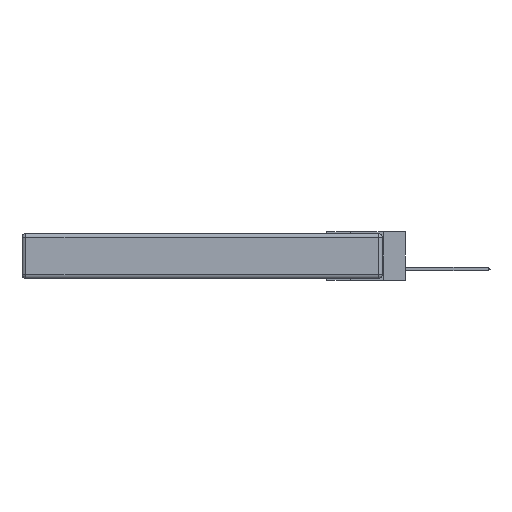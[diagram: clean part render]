
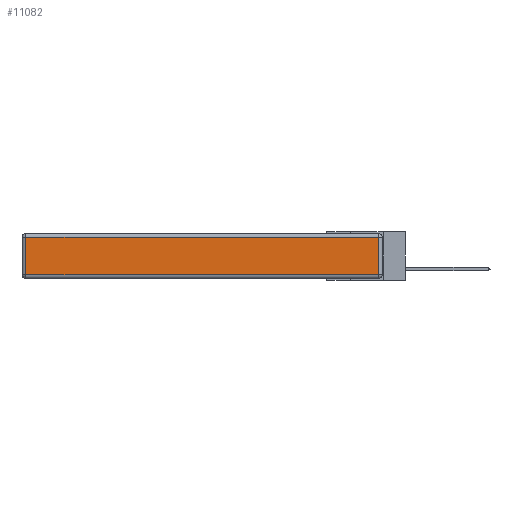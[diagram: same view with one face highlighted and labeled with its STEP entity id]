
A CAD part, left-side view. The second image highlights one B-rep face of the part: STEP entity #11082.
In plain terms, the highlighted planar face has unit normal (-1, 0, 0).
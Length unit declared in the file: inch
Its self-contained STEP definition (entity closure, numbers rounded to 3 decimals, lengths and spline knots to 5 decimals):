
#21 = EDGE_CURVE ( 'NONE', #5914, #2844, #9490, .T. ) ;
#1208 = ORIENTED_EDGE ( 'NONE', *, *, #21, .T. ) ;
#1388 = EDGE_CURVE ( 'NONE', #2844, #13567, #2982, .T. ) ;
#2119 = CARTESIAN_POINT ( 'NONE',  ( 0., 2.75, -0.03 ) ) ;
#2769 = DIRECTION ( 'NONE',  ( 0., 0., -1. ) ) ;
#2844 = VERTEX_POINT ( 'NONE', #3910 ) ;
#2982 = LINE ( 'NONE', #2119, #16490 ) ;
#3050 = DIRECTION ( 'NONE',  ( 0., -1., 0. ) ) ;
#3910 = CARTESIAN_POINT ( 'NONE',  ( 0., 0.03, -0.03 ) ) ;
#3968 = EDGE_CURVE ( 'NONE', #13567, #10532, #14343, .T. ) ;
#4058 = EDGE_CURVE ( 'NONE', #10532, #5914, #4957, .T. ) ;
#4348 = ORIENTED_EDGE ( 'NONE', *, *, #1388, .T. ) ;
#4957 = LINE ( 'NONE', #16259, #12901 ) ;
#5750 = DIRECTION ( 'NONE',  ( 0., 0., 1. ) ) ;
#5789 = DIRECTION ( 'NONE',  ( 0., 0., 1. ) ) ;
#5914 = VERTEX_POINT ( 'NONE', #15544 ) ;
#6654 = CARTESIAN_POINT ( 'NONE',  ( 0., 2.72, -0.343 ) ) ;
#7265 = CARTESIAN_POINT ( 'NONE',  ( 0., 2.72, -0.03 ) ) ;
#8497 = PLANE ( 'NONE',  #8661 ) ;
#8611 = DIRECTION ( 'NONE',  ( -1., 0., 0. ) ) ;
#8661 = AXIS2_PLACEMENT_3D ( 'NONE', #13619, #8611, #5789 ) ;
#9490 = LINE ( 'NONE', #16278, #13203 ) ;
#10532 = VERTEX_POINT ( 'NONE', #13823 ) ;
#11082 = ADVANCED_FACE ( 'NONE', ( #13714 ), #8497, .T. ) ;
#11393 = ORIENTED_EDGE ( 'NONE', *, *, #4058, .T. ) ;
#12901 = VECTOR ( 'NONE', #3050, 39.37008 ) ;
#13203 = VECTOR ( 'NONE', #5750, 39.37008 ) ;
#13567 = VERTEX_POINT ( 'NONE', #7265 ) ;
#13619 = CARTESIAN_POINT ( 'NONE',  ( 0., 0., -0.343 ) ) ;
#13714 = FACE_OUTER_BOUND ( 'NONE', #15087, .T. ) ;
#13782 = DIRECTION ( 'NONE',  ( 0., 1., 0. ) ) ;
#13823 = CARTESIAN_POINT ( 'NONE',  ( 0., 2.72, -0.313 ) ) ;
#14317 = VECTOR ( 'NONE', #2769, 39.37008 ) ;
#14343 = LINE ( 'NONE', #6654, #14317 ) ;
#14547 = ORIENTED_EDGE ( 'NONE', *, *, #3968, .T. ) ;
#15087 = EDGE_LOOP ( 'NONE', ( #11393, #1208, #4348, #14547 ) ) ;
#15544 = CARTESIAN_POINT ( 'NONE',  ( 0., 0.03, -0.313 ) ) ;
#16259 = CARTESIAN_POINT ( 'NONE',  ( 0., 0., -0.313 ) ) ;
#16278 = CARTESIAN_POINT ( 'NONE',  ( 0., 0.03, -0.343 ) ) ;
#16490 = VECTOR ( 'NONE', #13782, 39.37008 ) ;
